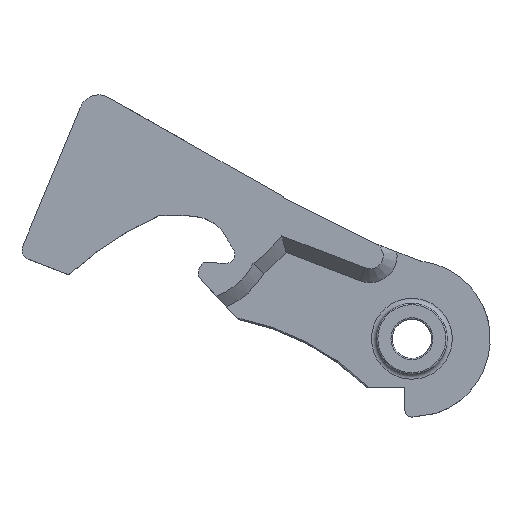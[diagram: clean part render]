
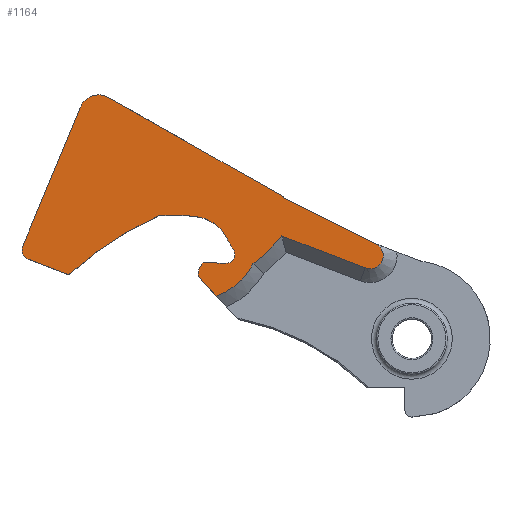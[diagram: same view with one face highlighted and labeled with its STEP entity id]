
A CAD part, top view. The second image highlights one B-rep face of the part: STEP entity #1164.
In plain terms, the highlighted planar face has unit normal (0, 0, 1).
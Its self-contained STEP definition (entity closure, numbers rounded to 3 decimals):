
#78=LINE('',#2034,#155);
#81=LINE('',#2042,#158);
#82=LINE('',#2046,#159);
#83=LINE('',#2066,#160);
#84=LINE('',#2072,#161);
#85=LINE('',#2076,#162);
#155=VECTOR('',#1532,10.);
#158=VECTOR('',#1539,10.);
#159=VECTOR('',#1542,10.);
#160=VECTOR('',#1561,10.);
#161=VECTOR('',#1566,10.);
#162=VECTOR('',#1569,10.);
#240=PLANE('',#1289);
#276=FACE_OUTER_BOUND('',#350,.T.);
#350=EDGE_LOOP('',(#889,#890,#891,#892,#893,#894,#895,#896,#897,#898,#899,
#900,#901,#902,#903,#904,#905,#906,#907,#908,#909));
#443=CIRCLE('',#1286,2.);
#444=CIRCLE('',#1290,1.);
#445=CIRCLE('',#1291,34.393);
#446=CIRCLE('',#1292,16.437);
#447=CIRCLE('',#1293,4.);
#448=CIRCLE('',#1294,15.);
#449=CIRCLE('',#1295,0.925);
#450=CIRCLE('',#1296,3.955);
#451=CIRCLE('',#1297,0.795);
#452=CIRCLE('',#1298,2.134);
#453=CIRCLE('',#1299,1.664);
#454=CIRCLE('',#1300,6.598);
#455=CIRCLE('',#1301,17.055);
#456=CIRCLE('',#1302,1.322);
#457=CIRCLE('',#1303,1.524);
#543=VERTEX_POINT('',#2027);
#544=VERTEX_POINT('',#2029);
#545=VERTEX_POINT('',#2033);
#548=VERTEX_POINT('',#2041);
#549=VERTEX_POINT('',#2043);
#550=VERTEX_POINT('',#2045);
#551=VERTEX_POINT('',#2047);
#552=VERTEX_POINT('',#2049);
#553=VERTEX_POINT('',#2051);
#554=VERTEX_POINT('',#2053);
#555=VERTEX_POINT('',#2055);
#556=VERTEX_POINT('',#2057);
#557=VERTEX_POINT('',#2059);
#558=VERTEX_POINT('',#2061);
#559=VERTEX_POINT('',#2063);
#560=VERTEX_POINT('',#2065);
#561=VERTEX_POINT('',#2067);
#562=VERTEX_POINT('',#2069);
#563=VERTEX_POINT('',#2071);
#564=VERTEX_POINT('',#2073);
#565=VERTEX_POINT('',#2075);
#674=EDGE_CURVE('',#543,#544,#443,.T.);
#676=EDGE_CURVE('',#544,#545,#78,.T.);
#680=EDGE_CURVE('',#543,#548,#81,.T.);
#681=EDGE_CURVE('',#549,#548,#444,.T.);
#682=EDGE_CURVE('',#549,#550,#82,.T.);
#683=EDGE_CURVE('',#550,#551,#445,.T.);
#684=EDGE_CURVE('',#551,#552,#446,.T.);
#685=EDGE_CURVE('',#552,#553,#447,.F.);
#686=EDGE_CURVE('',#554,#553,#448,.T.);
#687=EDGE_CURVE('',#554,#555,#449,.T.);
#688=EDGE_CURVE('',#555,#556,#450,.T.);
#689=EDGE_CURVE('',#556,#557,#451,.T.);
#690=EDGE_CURVE('',#557,#558,#452,.T.);
#691=EDGE_CURVE('',#558,#559,#453,.T.);
#692=EDGE_CURVE('',#559,#560,#83,.T.);
#693=EDGE_CURVE('',#560,#561,#454,.T.);
#694=EDGE_CURVE('',#561,#562,#455,.T.);
#695=EDGE_CURVE('',#563,#562,#84,.T.);
#696=EDGE_CURVE('',#564,#563,#456,.T.);
#697=EDGE_CURVE('',#564,#565,#85,.T.);
#698=EDGE_CURVE('',#565,#545,#457,.T.);
#889=ORIENTED_EDGE('',*,*,#674,.F.);
#890=ORIENTED_EDGE('',*,*,#680,.T.);
#891=ORIENTED_EDGE('',*,*,#681,.F.);
#892=ORIENTED_EDGE('',*,*,#682,.T.);
#893=ORIENTED_EDGE('',*,*,#683,.T.);
#894=ORIENTED_EDGE('',*,*,#684,.T.);
#895=ORIENTED_EDGE('',*,*,#685,.T.);
#896=ORIENTED_EDGE('',*,*,#686,.F.);
#897=ORIENTED_EDGE('',*,*,#687,.T.);
#898=ORIENTED_EDGE('',*,*,#688,.T.);
#899=ORIENTED_EDGE('',*,*,#689,.T.);
#900=ORIENTED_EDGE('',*,*,#690,.T.);
#901=ORIENTED_EDGE('',*,*,#691,.T.);
#902=ORIENTED_EDGE('',*,*,#692,.T.);
#903=ORIENTED_EDGE('',*,*,#693,.T.);
#904=ORIENTED_EDGE('',*,*,#694,.T.);
#905=ORIENTED_EDGE('',*,*,#695,.F.);
#906=ORIENTED_EDGE('',*,*,#696,.F.);
#907=ORIENTED_EDGE('',*,*,#697,.T.);
#908=ORIENTED_EDGE('',*,*,#698,.T.);
#909=ORIENTED_EDGE('',*,*,#676,.F.);
#1164=ADVANCED_FACE('',(#276),#240,.T.);
#1286=AXIS2_PLACEMENT_3D('',#2030,#1527,#1528);
#1289=AXIS2_PLACEMENT_3D('',#2040,#1537,#1538);
#1290=AXIS2_PLACEMENT_3D('',#2044,#1540,#1541);
#1291=AXIS2_PLACEMENT_3D('',#2048,#1543,#1544);
#1292=AXIS2_PLACEMENT_3D('',#2050,#1545,#1546);
#1293=AXIS2_PLACEMENT_3D('',#2052,#1547,#1548);
#1294=AXIS2_PLACEMENT_3D('',#2054,#1549,#1550);
#1295=AXIS2_PLACEMENT_3D('',#2056,#1551,#1552);
#1296=AXIS2_PLACEMENT_3D('',#2058,#1553,#1554);
#1297=AXIS2_PLACEMENT_3D('',#2060,#1555,#1556);
#1298=AXIS2_PLACEMENT_3D('',#2062,#1557,#1558);
#1299=AXIS2_PLACEMENT_3D('',#2064,#1559,#1560);
#1300=AXIS2_PLACEMENT_3D('',#2068,#1562,#1563);
#1301=AXIS2_PLACEMENT_3D('',#2070,#1564,#1565);
#1302=AXIS2_PLACEMENT_3D('',#2074,#1567,#1568);
#1303=AXIS2_PLACEMENT_3D('',#2077,#1570,#1571);
#1527=DIRECTION('center_axis',(0.,0.,-1.));
#1528=DIRECTION('ref_axis',(-0.324,0.946,0.));
#1532=DIRECTION('',(0.87,-0.494,0.));
#1537=DIRECTION('center_axis',(0.,0.,1.));
#1538=DIRECTION('ref_axis',(1.,0.,0.));
#1539=DIRECTION('',(-0.383,-0.924,0.));
#1540=DIRECTION('center_axis',(0.,0.,-1.));
#1541=DIRECTION('ref_axis',(-0.919,-0.394,0.));
#1542=DIRECTION('',(0.934,-0.358,0.));
#1543=DIRECTION('center_axis',(0.,0.,-1.));
#1544=DIRECTION('ref_axis',(0.41,-0.912,0.));
#1545=DIRECTION('center_axis',(0.,0.,-1.));
#1546=DIRECTION('ref_axis',(0.255,0.967,0.));
#1547=DIRECTION('center_axis',(0.,0.,1.));
#1548=DIRECTION('ref_axis',(-0.885,-0.466,0.));
#1549=DIRECTION('center_axis',(0.,0.,-1.));
#1550=DIRECTION('ref_axis',(-0.869,-0.494,0.));
#1551=DIRECTION('center_axis',(0.,0.,-1.));
#1552=DIRECTION('ref_axis',(-0.02,1.,0.));
#1553=DIRECTION('center_axis',(0.,0.,-1.));
#1554=DIRECTION('ref_axis',(0.204,0.979,0.));
#1555=DIRECTION('center_axis',(0.,0.,-1.));
#1556=DIRECTION('ref_axis',(0.387,0.922,0.));
#1557=DIRECTION('center_axis',(0.,0.,-1.));
#1558=DIRECTION('ref_axis',(0.215,0.977,0.));
#1559=DIRECTION('center_axis',(0.,0.,1.));
#1560=DIRECTION('ref_axis',(-0.654,0.757,0.));
#1561=DIRECTION('',(0.684,-0.729,0.));
#1562=DIRECTION('center_axis',(0.,0.,1.));
#1563=DIRECTION('ref_axis',(0.338,-0.941,0.));
#1564=DIRECTION('center_axis',(0.,0.,1.));
#1565=DIRECTION('ref_axis',(0.604,-0.797,0.));
#1566=DIRECTION('',(-0.934,0.358,0.));
#1567=DIRECTION('center_axis',(0.,0.,-1.));
#1568=DIRECTION('ref_axis',(0.358,0.934,0.));
#1569=DIRECTION('',(-0.895,0.445,0.));
#1570=DIRECTION('center_axis',(0.,0.,-1.));
#1571=DIRECTION('ref_axis',(0.934,-0.358,0.));
#2027=CARTESIAN_POINT('',(-33.346,23.302,3.813));
#2029=CARTESIAN_POINT('',(-30.511,24.275,3.813));
#2030=CARTESIAN_POINT('Origin',(-31.498,22.536,3.813));
#2033=CARTESIAN_POINT('',(-12.945,14.298,3.813));
#2034=CARTESIAN_POINT('',(-26.743,22.135,3.813));
#2040=CARTESIAN_POINT('Origin',(-25.059,13.756,3.813));
#2041=CARTESIAN_POINT('',(-39.147,9.325,3.813));
#2042=CARTESIAN_POINT('',(-34.108,21.466,3.813));
#2043=CARTESIAN_POINT('',(-38.582,8.008,3.813));
#2044=CARTESIAN_POINT('Origin',(-38.223,8.942,3.813));
#2045=CARTESIAN_POINT('',(-34.514,6.447,3.813));
#2046=CARTESIAN_POINT('',(-40.863,8.884,3.813));
#2047=CARTESIAN_POINT('',(-25.483,12.371,3.813));
#2048=CARTESIAN_POINT('Origin',(-11.369,-18.993,3.813));
#2049=CARTESIAN_POINT('',(-21.634,12.282,3.813));
#2050=CARTESIAN_POINT('Origin',(-23.936,-3.993,3.813));
#2051=CARTESIAN_POINT('',(-18.655,10.185,3.813));
#2052=CARTESIAN_POINT('Origin',(-22.194,8.321,3.813));
#2053=CARTESIAN_POINT('',(-17.962,9.002,3.813));
#2054=CARTESIAN_POINT('Origin',(-5.383,17.174,3.813));
#2055=CARTESIAN_POINT('',(-18.719,7.574,3.813));
#2056=CARTESIAN_POINT('Origin',(-18.737,8.498,3.813));
#2057=CARTESIAN_POINT('',(-19.765,7.65,3.813));
#2058=CARTESIAN_POINT('Origin',(-18.957,11.521,3.813));
#2059=CARTESIAN_POINT('',(-20.022,7.71,3.813));
#2060=CARTESIAN_POINT('Origin',(-19.715,8.444,3.813));
#2061=CARTESIAN_POINT('',(-20.941,7.71,3.813));
#2062=CARTESIAN_POINT('Origin',(-20.482,9.794,3.813));
#2063=CARTESIAN_POINT('',(-21.508,6.279,3.813));
#2064=CARTESIAN_POINT('Origin',(-19.853,6.451,3.813));
#2065=CARTESIAN_POINT('',(-19.65,4.297,3.813));
#2066=CARTESIAN_POINT('',(-21.508,6.279,3.813));
#2067=CARTESIAN_POINT('',(-15.987,7.542,3.813));
#2068=CARTESIAN_POINT('Origin',(-21.882,10.506,3.813));
#2069=CARTESIAN_POINT('',(-13.078,10.349,3.813));
#2070=CARTESIAN_POINT('Origin',(-26.29,21.133,3.813));
#2071=CARTESIAN_POINT('',(-4.688,7.128,3.813));
#2072=CARTESIAN_POINT('',(-4.688,7.128,3.813));
#2073=CARTESIAN_POINT('',(-3.74,9.598,3.813));
#2074=CARTESIAN_POINT('Origin',(-4.214,8.363,3.813));
#2075=CARTESIAN_POINT('',(-12.949,14.18,3.813));
#2076=CARTESIAN_POINT('',(-3.74,9.598,3.813));
#2077=CARTESIAN_POINT('Origin',(-11.425,14.18,3.813));
